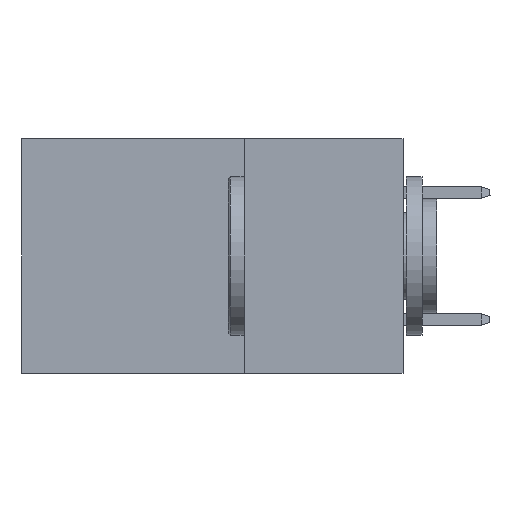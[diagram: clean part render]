
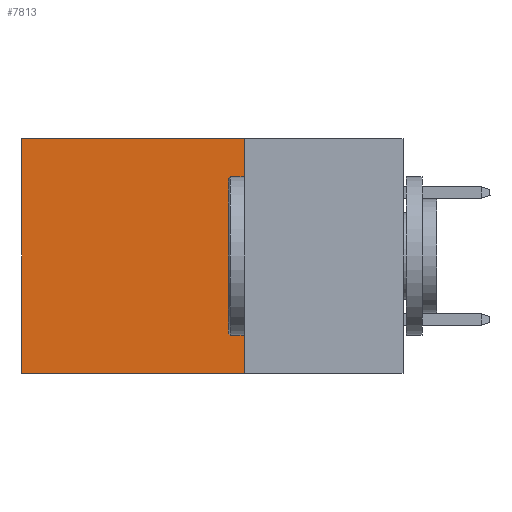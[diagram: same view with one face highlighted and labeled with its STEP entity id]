
A CAD part, left-side view. The second image highlights one B-rep face of the part: STEP entity #7813.
In plain terms, the highlighted planar face has unit normal (-1, 0, 0).
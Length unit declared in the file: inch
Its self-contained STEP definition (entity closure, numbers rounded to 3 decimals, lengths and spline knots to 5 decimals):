
#867 = LINE ( 'NONE', #14070, #11187 ) ;
#2703 = CARTESIAN_POINT ( 'NONE',  ( 0.2875, 0.25, 0. ) ) ;
#3342 = DIRECTION ( 'NONE',  ( 1., 0., 0. ) ) ;
#7251 = DIRECTION ( 'NONE',  ( 0., 1., 0. ) ) ;
#7813 = ADVANCED_FACE ( 'NONE', ( #42951 ), #16120, .F. ) ;
#8692 = VERTEX_POINT ( 'NONE', #31639 ) ;
#8749 = VERTEX_POINT ( 'NONE', #41076 ) ;
#11187 = VECTOR ( 'NONE', #27753, 39.37008 ) ;
#11481 = ORIENTED_EDGE ( 'NONE', *, *, #16036, .T. ) ;
#13792 = AXIS2_PLACEMENT_3D ( 'NONE', #2703, #3342, #43386 ) ;
#14070 = CARTESIAN_POINT ( 'NONE',  ( 0.2875, 0.6, 0. ) ) ;
#15440 = EDGE_CURVE ( 'NONE', #8749, #28461, #27024, .T. ) ;
#15564 = ORIENTED_EDGE ( 'NONE', *, *, #15440, .F. ) ;
#16036 = EDGE_CURVE ( 'NONE', #8692, #38838, #867, .T. ) ;
#16120 = PLANE ( 'NONE',  #13792 ) ;
#16907 = VECTOR ( 'NONE', #42630, 39.37008 ) ;
#18036 = CARTESIAN_POINT ( 'NONE',  ( 0.2875, 0.25, -0.37 ) ) ;
#19810 = EDGE_CURVE ( 'NONE', #28461, #38838, #31894, .T. ) ;
#20230 = LINE ( 'NONE', #37403, #40260 ) ;
#20690 = ORIENTED_EDGE ( 'NONE', *, *, #19810, .F. ) ;
#26577 = CARTESIAN_POINT ( 'NONE',  ( 0.2875, 0.25, -0.37 ) ) ;
#27024 = LINE ( 'NONE', #40445, #33676 ) ;
#27753 = DIRECTION ( 'NONE',  ( 0., 0., -1. ) ) ;
#28461 = VERTEX_POINT ( 'NONE', #18036 ) ;
#31639 = CARTESIAN_POINT ( 'NONE',  ( 0.2875, 0.6, 0. ) ) ;
#31894 = LINE ( 'NONE', #26577, #16907 ) ;
#33676 = VECTOR ( 'NONE', #37145, 39.37008 ) ;
#35409 = EDGE_CURVE ( 'NONE', #8749, #8692, #20230, .T. ) ;
#36444 = CARTESIAN_POINT ( 'NONE',  ( 0.2875, 0.6, -0.37 ) ) ;
#37145 = DIRECTION ( 'NONE',  ( 0., 0., -1. ) ) ;
#37403 = CARTESIAN_POINT ( 'NONE',  ( 0.2875, 0.25, 0. ) ) ;
#38838 = VERTEX_POINT ( 'NONE', #36444 ) ;
#39952 = EDGE_LOOP ( 'NONE', ( #11481, #20690, #15564, #40448 ) ) ;
#40260 = VECTOR ( 'NONE', #7251, 39.37008 ) ;
#40445 = CARTESIAN_POINT ( 'NONE',  ( 0.2875, 0.25, 0. ) ) ;
#40448 = ORIENTED_EDGE ( 'NONE', *, *, #35409, .T. ) ;
#41076 = CARTESIAN_POINT ( 'NONE',  ( 0.2875, 0.25, 0. ) ) ;
#42630 = DIRECTION ( 'NONE',  ( 0., 1., 0. ) ) ;
#42951 = FACE_OUTER_BOUND ( 'NONE', #39952, .T. ) ;
#43386 = DIRECTION ( 'NONE',  ( 0., 0., -1. ) ) ;
